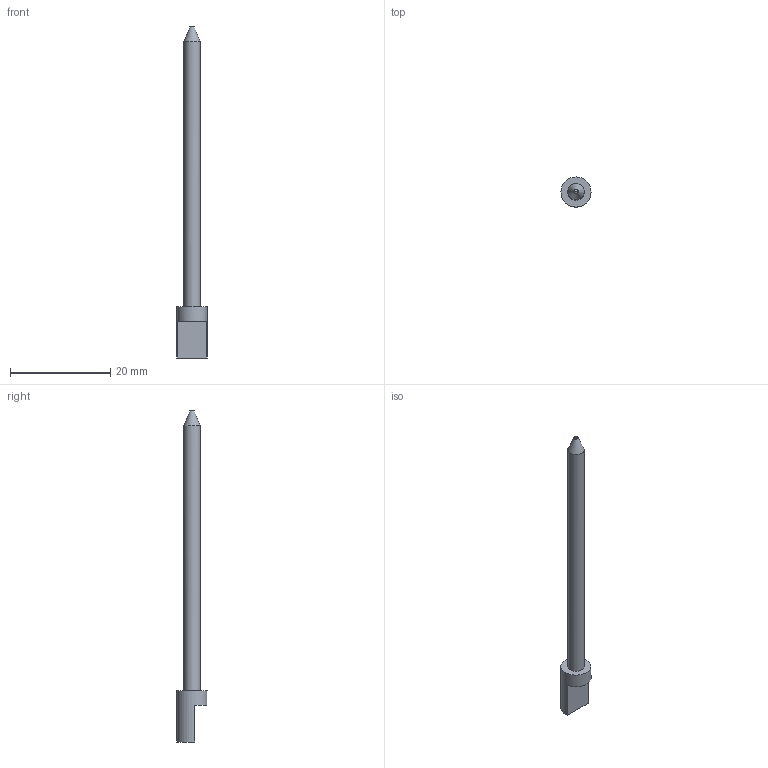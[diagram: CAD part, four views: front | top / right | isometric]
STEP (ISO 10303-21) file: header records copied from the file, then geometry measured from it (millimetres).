
FILE_DESCRIPTION(('FreeCAD Model'),'2;1');
FILE_NAME('AP9 simulated firing pin.step','2017-11-13T22:52:23',('Author'),(''), 'Open CASCADE STEP processor 6.8','FreeCAD','Unknown');
FILE_SCHEMA(('AUTOMOTIVE_DESIGN_CC2 { 1 2 10303 214 -1 1 5 4 }'));
Length unit declared in the file: millimetre
Products named in the file (1): Pocket
Bounding box: 6 x 6 x 66.2 mm (x, y, z)
Volume: 656 mm3; surface area: 783.1 mm2
Topology: 1 solids, 1 shells, 10 faces, 18 edges, 11 vertices
Faces by surface type: plane 5, cone 2, cylinder 2, bspline 1
Full cylindrical faces by diameter (mm): 3.25 x1, 6 x1
Entity records: 618 total; most frequent: CARTESIAN_POINT 242, DIRECTION 61, ORIENTED_EDGE 36, PCURVE 36, DEFINITIONAL_REPRESENTATION 36, LINE 26, VECTOR 26, EDGE_CURVE 18
